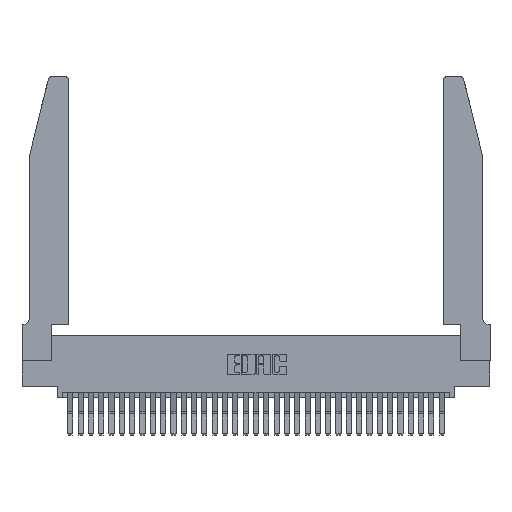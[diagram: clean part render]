
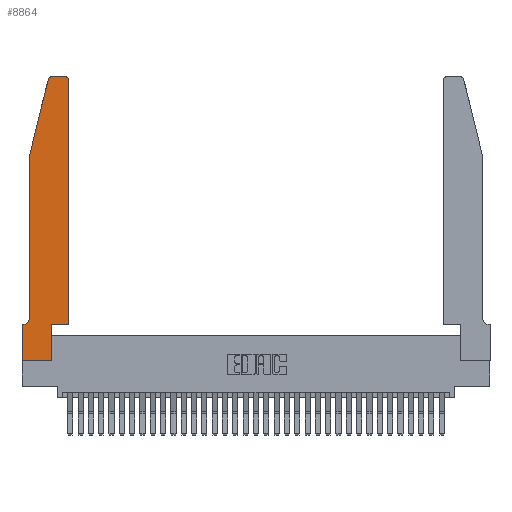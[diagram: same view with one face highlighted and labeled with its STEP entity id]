
A CAD part, top view. The second image highlights one B-rep face of the part: STEP entity #8864.
In plain terms, the highlighted planar face has unit normal (0, 0, 1).
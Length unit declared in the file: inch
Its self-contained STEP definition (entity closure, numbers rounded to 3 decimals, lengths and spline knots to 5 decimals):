
#70 = VERTEX_POINT ( 'NONE', #9941 ) ;
#325 = DIRECTION ( 'NONE',  ( 0., -1., 0. ) ) ;
#547 = VERTEX_POINT ( 'NONE', #28223 ) ;
#1087 = EDGE_CURVE ( 'NONE', #547, #24762, #25332, .T. ) ;
#1116 = CARTESIAN_POINT ( 'NONE',  ( 0.0755, 0.35, 0.37 ) ) ;
#1347 = VERTEX_POINT ( 'NONE', #26310 ) ;
#1918 = DIRECTION ( 'NONE',  ( 0., 0., -1. ) ) ;
#2405 = CARTESIAN_POINT ( 'NONE',  ( 0.284, 2.75, 0.37 ) ) ;
#2476 = VECTOR ( 'NONE', #34497, 39.37008 ) ;
#2894 = VERTEX_POINT ( 'NONE', #24795 ) ;
#3013 = DIRECTION ( 'NONE',  ( 0., 1., 0. ) ) ;
#3056 = DIRECTION ( 'NONE',  ( 1., 0., 0. ) ) ;
#3820 = CIRCLE ( 'NONE', #10635, 0.03 ) ;
#4020 = CARTESIAN_POINT ( 'NONE',  ( 0.2605, 2.75, 0.37 ) ) ;
#4961 = EDGE_CURVE ( 'NONE', #24762, #2894, #16134, .T. ) ;
#5423 = AXIS2_PLACEMENT_3D ( 'NONE', #26986, #27208, #22087 ) ;
#5812 = VERTEX_POINT ( 'NONE', #28453 ) ;
#6280 = VERTEX_POINT ( 'NONE', #34265 ) ;
#7088 = CARTESIAN_POINT ( 'NONE',  ( 0.0055, 0.42, 0.37 ) ) ;
#7134 = VECTOR ( 'NONE', #21225, 39.37008 ) ;
#8174 = EDGE_CURVE ( 'NONE', #29267, #5812, #24365, .T. ) ;
#8267 = CARTESIAN_POINT ( 'NONE',  ( 0.2865, 0.35, 0.37 ) ) ;
#8728 = LINE ( 'NONE', #32063, #31347 ) ;
#8776 = DIRECTION ( 'NONE',  ( 1., 0., 0. ) ) ;
#8864 = ADVANCED_FACE ( 'NONE', ( #30969 ), #18541, .T. ) ;
#9941 = CARTESIAN_POINT ( 'NONE',  ( 0.4505, 2.72, 0.37 ) ) ;
#10121 = EDGE_CURVE ( 'NONE', #2894, #18246, #17986, .T. ) ;
#10453 = CIRCLE ( 'NONE', #32934, 0.07 ) ;
#10635 = AXIS2_PLACEMENT_3D ( 'NONE', #32348, #19011, #3056 ) ;
#11111 = CARTESIAN_POINT ( 'NONE',  ( 0.284, 2.72, 0.37 ) ) ;
#11274 = LINE ( 'NONE', #32420, #25612 ) ;
#11748 = EDGE_CURVE ( 'NONE', #6280, #29267, #24211, .T. ) ;
#12761 = CARTESIAN_POINT ( 'NONE',  ( 0.4505, 0.35, 0.37 ) ) ;
#13601 = ORIENTED_EDGE ( 'NONE', *, *, #30254, .T. ) ;
#14704 = DIRECTION ( 'NONE',  ( -1., 0., 0. ) ) ;
#15501 = DIRECTION ( 'NONE',  ( -1., 0., 0. ) ) ;
#16134 = CIRCLE ( 'NONE', #18609, 0.03 ) ;
#16755 = CARTESIAN_POINT ( 'NONE',  ( 0., 0., 0.37 ) ) ;
#17986 = LINE ( 'NONE', #20580, #21379 ) ;
#18246 = VERTEX_POINT ( 'NONE', #32300 ) ;
#18541 = PLANE ( 'NONE',  #5423 ) ;
#18609 = AXIS2_PLACEMENT_3D ( 'NONE', #11111, #32567, #8776 ) ;
#19011 = DIRECTION ( 'NONE',  ( 0., 0., 1. ) ) ;
#19204 = VECTOR ( 'NONE', #24750, 39.37008 ) ;
#19548 = EDGE_CURVE ( 'NONE', #70, #547, #3820, .T. ) ;
#19991 = ORIENTED_EDGE ( 'NONE', *, *, #11748, .T. ) ;
#20111 = EDGE_CURVE ( 'NONE', #30069, #70, #26050, .T. ) ;
#20357 = EDGE_CURVE ( 'NONE', #27912, #24980, #11274, .T. ) ;
#20580 = CARTESIAN_POINT ( 'NONE',  ( 0.0755, 2., 0.37 ) ) ;
#21225 = DIRECTION ( 'NONE',  ( 0., 1., 0. ) ) ;
#21379 = VECTOR ( 'NONE', #23301, 39.37008 ) ;
#21729 = CARTESIAN_POINT ( 'NONE',  ( 0.2865, 0., 0.37 ) ) ;
#22087 = DIRECTION ( 'NONE',  ( 1., 0., 0. ) ) ;
#22800 = ORIENTED_EDGE ( 'NONE', *, *, #20111, .T. ) ;
#23301 = DIRECTION ( 'NONE',  ( -0.239, -0.971, 0. ) ) ;
#23767 = ORIENTED_EDGE ( 'NONE', *, *, #30061, .T. ) ;
#24211 = LINE ( 'NONE', #1116, #27064 ) ;
#24365 = LINE ( 'NONE', #29122, #2476 ) ;
#24578 = CARTESIAN_POINT ( 'NONE',  ( 0., 0.35, 0.37 ) ) ;
#24671 = ORIENTED_EDGE ( 'NONE', *, *, #28926, .T. ) ;
#24750 = DIRECTION ( 'NONE',  ( 1., 0., 0. ) ) ;
#24762 = VERTEX_POINT ( 'NONE', #2405 ) ;
#24795 = CARTESIAN_POINT ( 'NONE',  ( 0.25487, 2.72718, 0.37 ) ) ;
#24980 = VERTEX_POINT ( 'NONE', #8267 ) ;
#25332 = LINE ( 'NONE', #4020, #32391 ) ;
#25540 = LINE ( 'NONE', #30062, #19204 ) ;
#25612 = VECTOR ( 'NONE', #3013, 39.37008 ) ;
#26050 = LINE ( 'NONE', #12761, #7134 ) ;
#26310 = CARTESIAN_POINT ( 'NONE',  ( 0.0755, 0.42, 0.37 ) ) ;
#26681 = ORIENTED_EDGE ( 'NONE', *, *, #1087, .T. ) ;
#26986 = CARTESIAN_POINT ( 'NONE',  ( 0., 0.35, 0.37 ) ) ;
#27064 = VECTOR ( 'NONE', #14704, 39.37008 ) ;
#27208 = DIRECTION ( 'NONE',  ( 0., 0., 1. ) ) ;
#27912 = VERTEX_POINT ( 'NONE', #21729 ) ;
#28179 = DIRECTION ( 'NONE',  ( -1., 0., 0. ) ) ;
#28223 = CARTESIAN_POINT ( 'NONE',  ( 0.4205, 2.75, 0.37 ) ) ;
#28453 = CARTESIAN_POINT ( 'NONE',  ( 0., 0., 0.37 ) ) ;
#28926 = EDGE_CURVE ( 'NONE', #1347, #6280, #10453, .T. ) ;
#28971 = ORIENTED_EDGE ( 'NONE', *, *, #8174, .T. ) ;
#29122 = CARTESIAN_POINT ( 'NONE',  ( 0., 0., 0.37 ) ) ;
#29145 = EDGE_LOOP ( 'NONE', ( #26681, #32667, #29821, #23767, #24671, #19991, #28971, #29501, #34187, #13601, #22800, #32048 ) ) ;
#29267 = VERTEX_POINT ( 'NONE', #24578 ) ;
#29501 = ORIENTED_EDGE ( 'NONE', *, *, #34639, .T. ) ;
#29821 = ORIENTED_EDGE ( 'NONE', *, *, #10121, .T. ) ;
#30061 = EDGE_CURVE ( 'NONE', #18246, #1347, #8728, .T. ) ;
#30062 = CARTESIAN_POINT ( 'NONE',  ( 0.4505, 0.35, 0.37 ) ) ;
#30069 = VERTEX_POINT ( 'NONE', #32525 ) ;
#30217 = DIRECTION ( 'NONE',  ( 1., 0., 0. ) ) ;
#30254 = EDGE_CURVE ( 'NONE', #24980, #30069, #25540, .T. ) ;
#30619 = LINE ( 'NONE', #16755, #34019 ) ;
#30969 = FACE_OUTER_BOUND ( 'NONE', #29145, .T. ) ;
#31347 = VECTOR ( 'NONE', #325, 39.37008 ) ;
#32048 = ORIENTED_EDGE ( 'NONE', *, *, #19548, .T. ) ;
#32063 = CARTESIAN_POINT ( 'NONE',  ( 0.0755, 2., 0.37 ) ) ;
#32300 = CARTESIAN_POINT ( 'NONE',  ( 0.0755, 2., 0.37 ) ) ;
#32348 = CARTESIAN_POINT ( 'NONE',  ( 0.4205, 2.72, 0.37 ) ) ;
#32391 = VECTOR ( 'NONE', #28179, 39.37008 ) ;
#32420 = CARTESIAN_POINT ( 'NONE',  ( 0.2865, 0.35, 0.37 ) ) ;
#32525 = CARTESIAN_POINT ( 'NONE',  ( 0.4505, 0.35, 0.37 ) ) ;
#32567 = DIRECTION ( 'NONE',  ( 0., 0., 1. ) ) ;
#32667 = ORIENTED_EDGE ( 'NONE', *, *, #4961, .T. ) ;
#32934 = AXIS2_PLACEMENT_3D ( 'NONE', #7088, #1918, #15501 ) ;
#34019 = VECTOR ( 'NONE', #30217, 39.37008 ) ;
#34187 = ORIENTED_EDGE ( 'NONE', *, *, #20357, .T. ) ;
#34265 = CARTESIAN_POINT ( 'NONE',  ( 0.0055, 0.35, 0.37 ) ) ;
#34497 = DIRECTION ( 'NONE',  ( 0., -1., 0. ) ) ;
#34639 = EDGE_CURVE ( 'NONE', #5812, #27912, #30619, .T. ) ;
